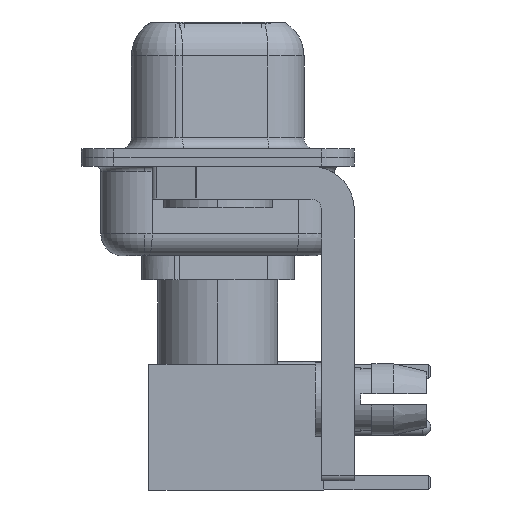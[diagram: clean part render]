
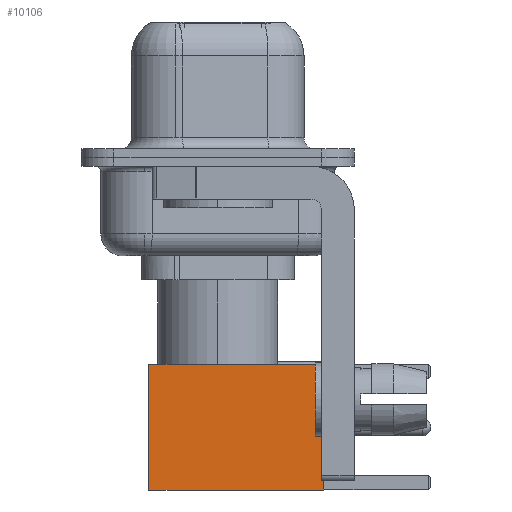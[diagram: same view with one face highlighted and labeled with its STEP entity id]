
A CAD part, left-side view. The second image highlights one B-rep face of the part: STEP entity #10106.
In plain terms, the highlighted face is planar.
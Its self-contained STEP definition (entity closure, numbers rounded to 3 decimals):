
#341 = LINE ( 'NONE', #14258, #10980 ) ;
#1846 = CARTESIAN_POINT ( 'NONE',  ( 2.875, 2.875, 0. ) ) ;
#2763 = ORIENTED_EDGE ( 'NONE', *, *, #10052, .T. ) ;
#4151 = DIRECTION ( 'NONE',  ( 0., 0., -1. ) ) ;
#4232 = DIRECTION ( 'NONE',  ( -1., 0., 0. ) ) ;
#4481 = VECTOR ( 'NONE', #4151, 1000. ) ;
#5972 = ORIENTED_EDGE ( 'NONE', *, *, #26618, .F. ) ;
#6167 = CARTESIAN_POINT ( 'NONE',  ( 2.875, 2.875, 0. ) ) ;
#6249 = VERTEX_POINT ( 'NONE', #25564 ) ;
#6476 = VERTEX_POINT ( 'NONE', #6167 ) ;
#6914 = LINE ( 'NONE', #13705, #4481 ) ;
#8398 = EDGE_CURVE ( 'NONE', #10244, #29293, #341, .T. ) ;
#9085 = CARTESIAN_POINT ( 'NONE',  ( -2.875, 2.875, 8. ) ) ;
#10052 = EDGE_CURVE ( 'NONE', #6476, #6249, #25420, .T. ) ;
#10106 = ADVANCED_FACE ( 'NONE', ( #29618 ), #15977, .T. ) ;
#10244 = VERTEX_POINT ( 'NONE', #16598 ) ;
#10980 = VECTOR ( 'NONE', #21687, 1000. ) ;
#11019 = DIRECTION ( 'NONE',  ( 0., 1., 0. ) ) ;
#13443 = LINE ( 'NONE', #1846, #30042 ) ;
#13660 = ORIENTED_EDGE ( 'NONE', *, *, #8398, .F. ) ;
#13705 = CARTESIAN_POINT ( 'NONE',  ( -2.875, 2.875, 0. ) ) ;
#14258 = CARTESIAN_POINT ( 'NONE',  ( 0., 2.875, 8. ) ) ;
#14621 = EDGE_CURVE ( 'NONE', #10244, #6476, #13443, .T. ) ;
#15977 = PLANE ( 'NONE',  #16956 ) ;
#16598 = CARTESIAN_POINT ( 'NONE',  ( 2.875, 2.875, 8. ) ) ;
#16956 = AXIS2_PLACEMENT_3D ( 'NONE', #27744, #11019, #22782 ) ;
#18576 = DIRECTION ( 'NONE',  ( 0., 0., -1. ) ) ;
#20604 = EDGE_LOOP ( 'NONE', ( #28240, #2763, #5972, #13660 ) ) ;
#21398 = VECTOR ( 'NONE', #4232, 1000. ) ;
#21687 = DIRECTION ( 'NONE',  ( -1., 0., 0. ) ) ;
#22782 = DIRECTION ( 'NONE',  ( 0., 0., 1. ) ) ;
#25420 = LINE ( 'NONE', #29771, #21398 ) ;
#25564 = CARTESIAN_POINT ( 'NONE',  ( -2.875, 2.875, 0. ) ) ;
#26618 = EDGE_CURVE ( 'NONE', #29293, #6249, #6914, .T. ) ;
#27744 = CARTESIAN_POINT ( 'NONE',  ( 2.875, 2.875, 0. ) ) ;
#28240 = ORIENTED_EDGE ( 'NONE', *, *, #14621, .T. ) ;
#29293 = VERTEX_POINT ( 'NONE', #9085 ) ;
#29618 = FACE_OUTER_BOUND ( 'NONE', #20604, .T. ) ;
#29771 = CARTESIAN_POINT ( 'NONE',  ( 0., 2.875, 0. ) ) ;
#30042 = VECTOR ( 'NONE', #18576, 1000. ) ;
